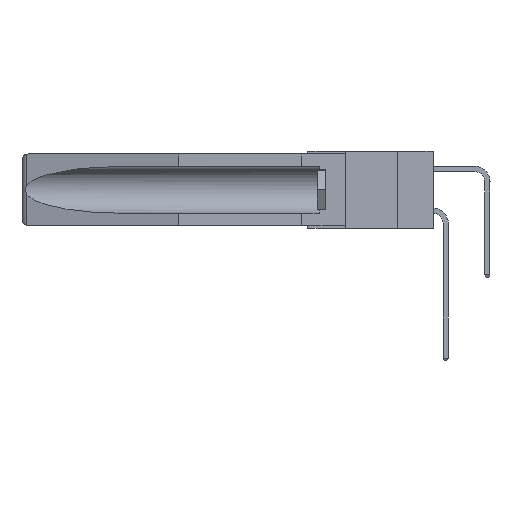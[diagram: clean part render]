
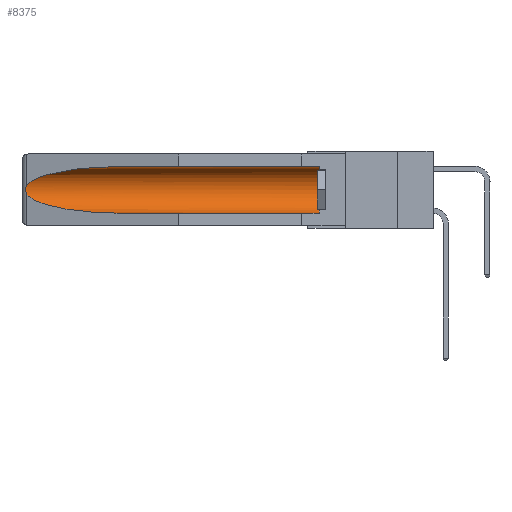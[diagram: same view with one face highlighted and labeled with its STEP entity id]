
A CAD part, left-side view. The second image highlights one B-rep face of the part: STEP entity #8375.
In plain terms, the highlighted cylindrical face has radius 2.857 mm (diameter 5.715 mm), a partial arc.
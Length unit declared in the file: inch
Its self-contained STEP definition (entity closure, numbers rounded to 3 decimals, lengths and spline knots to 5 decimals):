
#42 = VERTEX_POINT ( 'NONE', #14403 ) ;
#135 = VERTEX_POINT ( 'NONE', #7934 ) ;
#538 = CARTESIAN_POINT ( 'NONE',  ( 0.26597, 1.52961, -0.15275 ) ) ;
#839 = EDGE_CURVE ( 'NONE', #42, #3700, #18157, .T. ) ;
#905 = CARTESIAN_POINT ( 'NONE',  ( 0.21114, 1.30732, -0.059 ) ) ;
#1554 = DIRECTION ( 'NONE',  ( 0., 1., 0. ) ) ;
#2004 = CARTESIAN_POINT ( 'NONE',  ( 0.2673, 1.53269, -0.17917 ) ) ;
#2248 = CARTESIAN_POINT ( 'NONE',  ( 0.155, 1.07973, -0.059 ) ) ;
#2298 = CARTESIAN_POINT ( 'NONE',  ( 0.155, 1.07973, -0.284 ) ) ;
#2872 = CARTESIAN_POINT ( 'NONE',  ( 0.155, -0.30754, -0.284 ) ) ;
#3539 = CARTESIAN_POINT ( 'NONE',  ( 0.2675, 1.53308, -0.16763 ) ) ;
#3700 = VERTEX_POINT ( 'NONE', #2248 ) ;
#3778 = CARTESIAN_POINT ( 'NONE',  ( 0.21114, 1.30732, -0.284 ) ) ;
#4141 = VERTEX_POINT ( 'NONE', #8345 ) ;
#4628 = ORIENTED_EDGE ( 'NONE', *, *, #839, .T. ) ;
#5167 = CARTESIAN_POINT ( 'NONE',  ( 0.26537, 1.52718, -0.14972 ) ) ;
#6297 = EDGE_CURVE ( 'NONE', #10307, #8724, #7636, .T. ) ;
#6773 = CARTESIAN_POINT ( 'NONE',  ( 0.155, -0.30754, -0.059 ) ) ;
#6798 = CARTESIAN_POINT ( 'NONE',  ( 0.2673, 1.5327, -0.16383 ) ) ;
#7003 = CARTESIAN_POINT ( 'NONE',  ( 0.26597, 1.5296, -0.19026 ) ) ;
#7086 = CARTESIAN_POINT ( 'NONE',  ( 0.25451, 1.48313, -0.24835 ) ) ;
#7636 = B_SPLINE_CURVE_WITH_KNOTS ( 'NONE', 3,
 ( #5167, #538, #19802, #6798, #3539, #10067, #2004, #18028, #7003, #8425 ),
 .UNSPECIFIED., .F., .F.,
 ( 4, 2, 2, 2, 4 ),
 ( 0., 0.00029, 0.00058, 0.00087, 0.00117 ),
 .UNSPECIFIED. ) ;
#7666 = EDGE_CURVE ( 'NONE', #4141, #42, #14864, .T. ) ;
#7934 = CARTESIAN_POINT ( 'NONE',  ( 0.155, 1.07973, -0.284 ) ) ;
#8285 = FACE_OUTER_BOUND ( 'NONE', #18231, .T. ) ;
#8345 = CARTESIAN_POINT ( 'NONE',  ( 0.155, 0.126, -0.284 ) ) ;
#8371 = AXIS2_PLACEMENT_3D ( 'NONE', #13112, #11648, #11585 ) ;
#8375 = ADVANCED_FACE ( 'NONE', ( #8285 ), #9325, .F. ) ;
#8425 = CARTESIAN_POINT ( 'NONE',  ( 0.26537, 1.52718, -0.19328 ) ) ;
#8724 = VERTEX_POINT ( 'NONE', #17146 ) ;
#8861 = VECTOR ( 'NONE', #1554, 39.37008 ) ;
#9325 = CYLINDRICAL_SURFACE ( 'NONE', #17079, 0.1125 ) ;
#9518 = ORIENTED_EDGE ( 'NONE', *, *, #16075, .T. ) ;
#10067 = CARTESIAN_POINT ( 'NONE',  ( 0.2675, 1.53308, -0.17534 ) ) ;
#10307 = VERTEX_POINT ( 'NONE', #12556 ) ;
#10591 = CARTESIAN_POINT ( 'NONE',  ( 0.155, 1.07973, -0.059 ) ) ;
#10953 = DIRECTION ( 'NONE',  ( 0., 1., 0. ) ) ;
#11170 =( BOUNDED_CURVE ( )  B_SPLINE_CURVE ( 3, ( #13641, #7086, #3778, #2298 ),
 .UNSPECIFIED., .F., .F. ) 
 B_SPLINE_CURVE_WITH_KNOTS ( ( 4, 4 ),
 ( 0.1948, 1.5708 ),
 .UNSPECIFIED. ) 
 CURVE ( )  GEOMETRIC_REPRESENTATION_ITEM ( )  RATIONAL_B_SPLINE_CURVE ( ( 1., 0.848, 0.848, 1. ) ) 
 REPRESENTATION_ITEM ( '' )  );
#11585 = DIRECTION ( 'NONE',  ( 0., 0., 1. ) ) ;
#11648 = DIRECTION ( 'NONE',  ( 0., -1., 0. ) ) ;
#11821 = EDGE_CURVE ( 'NONE', #4141, #135, #15085, .T. ) ;
#11894 = CARTESIAN_POINT ( 'NONE',  ( 0.25451, 1.48313, -0.09465 ) ) ;
#12556 = CARTESIAN_POINT ( 'NONE',  ( 0.26537, 1.52718, -0.14972 ) ) ;
#13112 = CARTESIAN_POINT ( 'NONE',  ( 0.155, 0.126, -0.1715 ) ) ;
#13641 = CARTESIAN_POINT ( 'NONE',  ( 0.26537, 1.52718, -0.19328 ) ) ;
#13845 = VECTOR ( 'NONE', #10953, 39.37008 ) ;
#14403 = CARTESIAN_POINT ( 'NONE',  ( 0.155, 0.126, -0.059 ) ) ;
#14760 = ORIENTED_EDGE ( 'NONE', *, *, #14977, .T. ) ;
#14768 = ORIENTED_EDGE ( 'NONE', *, *, #11821, .F. ) ;
#14864 = CIRCLE ( 'NONE', #8371, 0.1125 ) ;
#14977 = EDGE_CURVE ( 'NONE', #3700, #10307, #19503, .T. ) ;
#15041 = CARTESIAN_POINT ( 'NONE',  ( 0.155, -0.30754, -0.1715 ) ) ;
#15085 = LINE ( 'NONE', #2872, #13845 ) ;
#15112 = CARTESIAN_POINT ( 'NONE',  ( 0.26537, 1.52718, -0.14972 ) ) ;
#16075 = EDGE_CURVE ( 'NONE', #8724, #135, #11170, .T. ) ;
#16634 = ORIENTED_EDGE ( 'NONE', *, *, #6297, .T. ) ;
#16635 = DIRECTION ( 'NONE',  ( 0., 1., 0. ) ) ;
#17079 = AXIS2_PLACEMENT_3D ( 'NONE', #15041, #16635, #19916 ) ;
#17146 = CARTESIAN_POINT ( 'NONE',  ( 0.26537, 1.52718, -0.19328 ) ) ;
#17739 = ORIENTED_EDGE ( 'NONE', *, *, #7666, .T. ) ;
#18028 = CARTESIAN_POINT ( 'NONE',  ( 0.26655, 1.53094, -0.18657 ) ) ;
#18157 = LINE ( 'NONE', #6773, #8861 ) ;
#18231 = EDGE_LOOP ( 'NONE', ( #14760, #16634, #9518, #14768, #17739, #4628 ) ) ;
#19503 =( BOUNDED_CURVE ( )  B_SPLINE_CURVE ( 3, ( #10591, #905, #11894, #15112 ),
 .UNSPECIFIED., .F., .F. ) 
 B_SPLINE_CURVE_WITH_KNOTS ( ( 4, 4 ),
 ( 4.71239, 6.08839 ),
 .UNSPECIFIED. ) 
 CURVE ( )  GEOMETRIC_REPRESENTATION_ITEM ( )  RATIONAL_B_SPLINE_CURVE ( ( 1., 0.848, 0.848, 1. ) ) 
 REPRESENTATION_ITEM ( '' )  );
#19802 = CARTESIAN_POINT ( 'NONE',  ( 0.26654, 1.53092, -0.15636 ) ) ;
#19916 = DIRECTION ( 'NONE',  ( 0., 0., 1. ) ) ;
